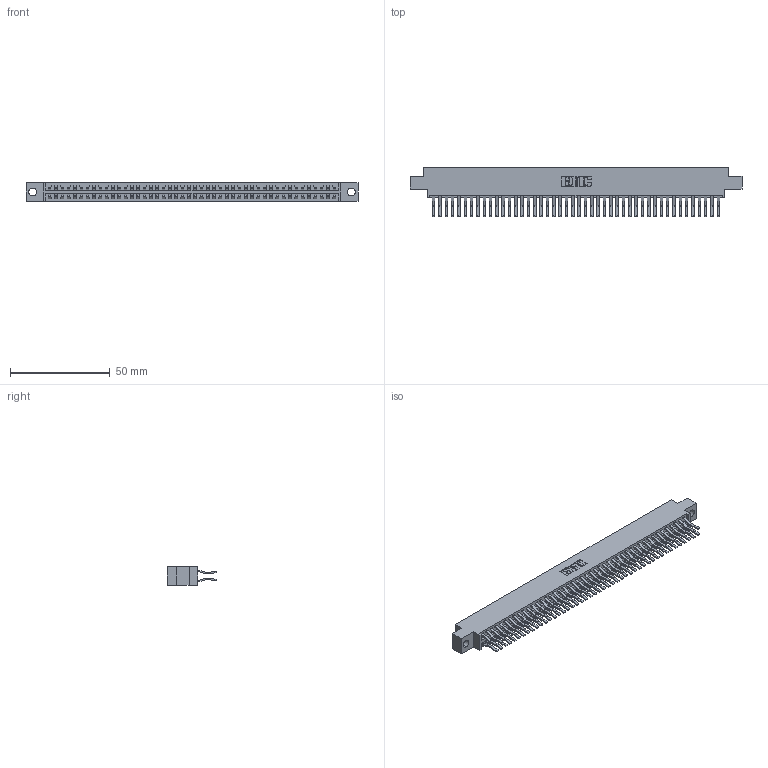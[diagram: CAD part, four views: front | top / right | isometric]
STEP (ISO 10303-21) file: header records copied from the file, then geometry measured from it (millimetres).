
FILE_DESCRIPTION (( 'STEP AP203' ), '1' );
FILE_NAME ('346-092-560-804.STEP', '2022-05-26T08:53:46', ( '' ), ( '' ), 'SwSTEP 2.0', 'SolidWorks 2020', '' );
FILE_SCHEMA (( 'CONFIG_CONTROL_DESIGN' ));
Length unit declared in the file: inch
Products named in the file (3): 346-092-560-804; 346 Part_0.170 Offset - 0.156 Dia-TH; 345-292-001_560 Tail
Assembly tree (93 placements, depth 2):
  346-092-560-804
    346 Part_0.170 Offset - 0.156 Dia-TH
    345-292-001_560 Tail  x92
Bounding box: 166.62 x 24.78 x 9.4 mm (x, y, z)
Volume: 16621.4 mm3; surface area: 24546.5 mm2
Topology: 93 solids, 93 shells, 5108 faces, 15189 edges, 10002 vertices
Faces by surface type: plane 3314, cylinder 1794
Entity records: 30121 total; most frequent: CARTESIAN_POINT 4966, ORIENTED_EDGE 4898, DIRECTION 4429, EDGE_CURVE 2449, LINE 2129, VECTOR 2129, VERTEX_POINT 1630, AXIS2_PLACEMENT_3D 1150
